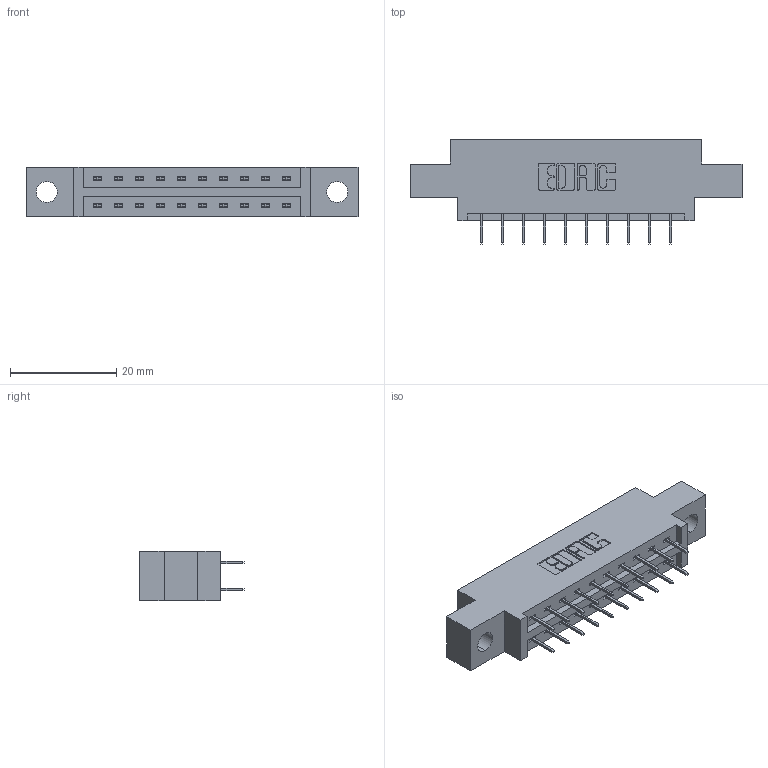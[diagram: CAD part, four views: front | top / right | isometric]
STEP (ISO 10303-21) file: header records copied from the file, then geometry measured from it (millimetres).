
FILE_DESCRIPTION (( 'STEP AP203' ), '1' );
FILE_NAME ('337-020-524-804.STEP', '2018-08-05T08:59:46', ( '' ), ( '' ), 'SwSTEP 2.0', 'SolidWorks 2016', '' );
FILE_SCHEMA (( 'CONFIG_CONTROL_DESIGN' ));
Length unit declared in the file: inch
Products named in the file (3): 337-020-524-804; 337 Part_0.170 Offset - 0.156 Dia-TH; 345-292-001_345-293-124
Assembly tree (21 placements, depth 2):
  337-020-524-804
    337 Part_0.170 Offset - 0.156 Dia-TH
    345-292-001_345-293-124  x20
Bounding box: 62.64 x 19.69 x 9.4 mm (x, y, z)
Volume: 5939.5 mm3; surface area: 6215.3 mm2
Topology: 21 solids, 21 shells, 1278 faces, 3623 edges, 2334 vertices
Faces by surface type: plane 954, cylinder 324
Entity records: 12101 total; most frequent: CARTESIAN_POINT 2066, ORIENTED_EDGE 2002, DIRECTION 1817, EDGE_CURVE 1001, LINE 877, VECTOR 877, VERTEX_POINT 662, AXIS2_PLACEMENT_3D 470
